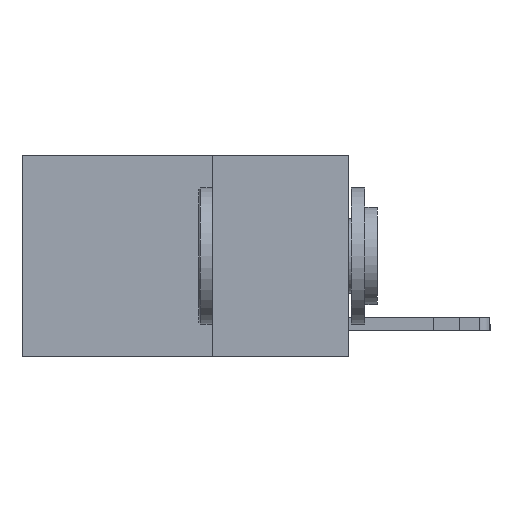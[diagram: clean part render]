
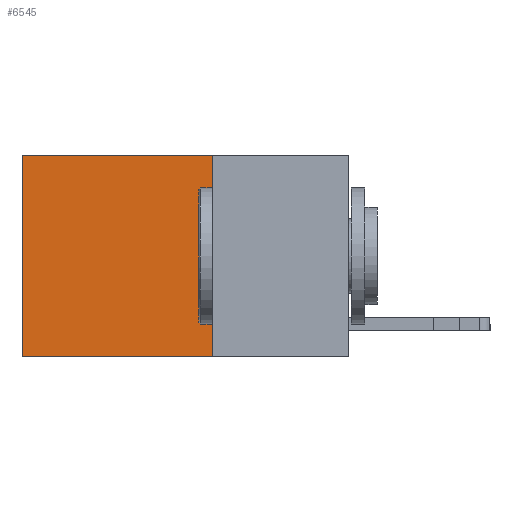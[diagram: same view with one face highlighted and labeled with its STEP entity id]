
A CAD part, left-side view. The second image highlights one B-rep face of the part: STEP entity #6545.
In plain terms, the highlighted planar face has unit normal (-1, 0, 0).
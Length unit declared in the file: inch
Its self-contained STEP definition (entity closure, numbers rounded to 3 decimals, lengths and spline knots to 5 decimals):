
#221 = DIRECTION ( 'NONE',  ( 0., 0., -1. ) ) ;
#792 = EDGE_CURVE ( 'NONE', #12915, #9845, #11108, .T. ) ;
#1132 = EDGE_CURVE ( 'NONE', #17842, #15348, #4007, .T. ) ;
#2618 = ORIENTED_EDGE ( 'NONE', *, *, #19872, .F. ) ;
#2639 = DIRECTION ( 'NONE',  ( 0., 0., -1. ) ) ;
#2690 = CARTESIAN_POINT ( 'NONE',  ( 0.2625, 0.6, 0. ) ) ;
#3145 = VECTOR ( 'NONE', #221, 39.37008 ) ;
#3283 = PLANE ( 'NONE',  #20358 ) ;
#3733 = ORIENTED_EDGE ( 'NONE', *, *, #5057, .T. ) ;
#4007 = LINE ( 'NONE', #8995, #20563 ) ;
#5057 = EDGE_CURVE ( 'NONE', #9845, #15348, #12018, .T. ) ;
#5870 = ORIENTED_EDGE ( 'NONE', *, *, #792, .T. ) ;
#6492 = DIRECTION ( 'NONE',  ( 0., 0., -1. ) ) ;
#6545 = ADVANCED_FACE ( 'NONE', ( #10123 ), #3283, .F. ) ;
#7503 = LINE ( 'NONE', #15976, #18552 ) ;
#7740 = CARTESIAN_POINT ( 'NONE',  ( 0.2625, 0.25, -0.37 ) ) ;
#8995 = CARTESIAN_POINT ( 'NONE',  ( 0.2625, 0.25, -0.37 ) ) ;
#9457 = DIRECTION ( 'NONE',  ( 0., 1., 0. ) ) ;
#9845 = VERTEX_POINT ( 'NONE', #2690 ) ;
#9909 = CARTESIAN_POINT ( 'NONE',  ( 0.2625, 0.25, 0. ) ) ;
#10123 = FACE_OUTER_BOUND ( 'NONE', #16748, .T. ) ;
#10819 = CARTESIAN_POINT ( 'NONE',  ( 0.2625, 0.6, -0.37 ) ) ;
#11108 = LINE ( 'NONE', #17812, #17733 ) ;
#12018 = LINE ( 'NONE', #15414, #3145 ) ;
#12593 = ORIENTED_EDGE ( 'NONE', *, *, #1132, .F. ) ;
#12915 = VERTEX_POINT ( 'NONE', #13288 ) ;
#13288 = CARTESIAN_POINT ( 'NONE',  ( 0.2625, 0.25, 0. ) ) ;
#15348 = VERTEX_POINT ( 'NONE', #10819 ) ;
#15414 = CARTESIAN_POINT ( 'NONE',  ( 0.2625, 0.6, 0. ) ) ;
#15976 = CARTESIAN_POINT ( 'NONE',  ( 0.2625, 0.25, 0. ) ) ;
#16748 = EDGE_LOOP ( 'NONE', ( #3733, #12593, #2618, #5870 ) ) ;
#17733 = VECTOR ( 'NONE', #9457, 39.37008 ) ;
#17812 = CARTESIAN_POINT ( 'NONE',  ( 0.2625, 0.25, 0. ) ) ;
#17842 = VERTEX_POINT ( 'NONE', #7740 ) ;
#18552 = VECTOR ( 'NONE', #2639, 39.37008 ) ;
#19872 = EDGE_CURVE ( 'NONE', #12915, #17842, #7503, .T. ) ;
#20358 = AXIS2_PLACEMENT_3D ( 'NONE', #9909, #21604, #6492 ) ;
#20563 = VECTOR ( 'NONE', #20781, 39.37008 ) ;
#20781 = DIRECTION ( 'NONE',  ( 0., 1., 0. ) ) ;
#21604 = DIRECTION ( 'NONE',  ( 1., 0., 0. ) ) ;
